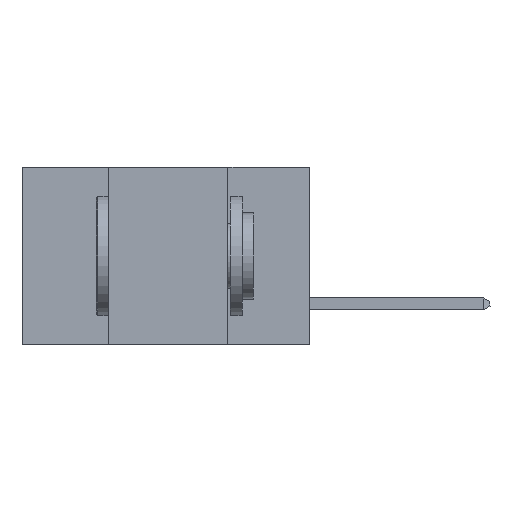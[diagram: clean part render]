
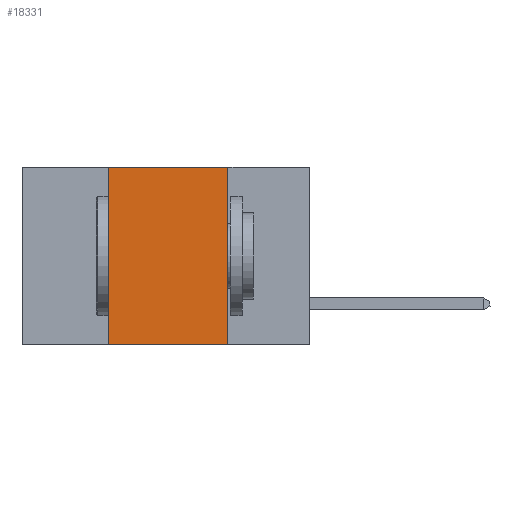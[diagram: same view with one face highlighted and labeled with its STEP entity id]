
A CAD part, left-side view. The second image highlights one B-rep face of the part: STEP entity #18331.
In plain terms, the highlighted planar face has unit normal (-1, 0, 0).
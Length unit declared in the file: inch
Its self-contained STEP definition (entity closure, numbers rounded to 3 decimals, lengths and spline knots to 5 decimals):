
#239 = VECTOR ( 'NONE', #10059, 39.37008 ) ;
#718 = VERTEX_POINT ( 'NONE', #21697 ) ;
#831 = EDGE_LOOP ( 'NONE', ( #9684, #24797, #4536, #24205 ) ) ;
#2341 = FACE_OUTER_BOUND ( 'NONE', #831, .T. ) ;
#3418 = EDGE_CURVE ( 'NONE', #30850, #718, #31739, .T. ) ;
#4372 = VECTOR ( 'NONE', #29341, 39.37008 ) ;
#4536 = ORIENTED_EDGE ( 'NONE', *, *, #8881, .F. ) ;
#5745 = CARTESIAN_POINT ( 'NONE',  ( 0., 0.42, 0. ) ) ;
#6669 = CARTESIAN_POINT ( 'NONE',  ( 0., 0.17, 0. ) ) ;
#6925 = LINE ( 'NONE', #30030, #239 ) ;
#7791 = PLANE ( 'NONE',  #30682 ) ;
#8881 = EDGE_CURVE ( 'NONE', #30850, #23092, #17730, .T. ) ;
#9241 = CARTESIAN_POINT ( 'NONE',  ( 0., 0.42, 0. ) ) ;
#9684 = ORIENTED_EDGE ( 'NONE', *, *, #11630, .F. ) ;
#10059 = DIRECTION ( 'NONE',  ( 0., 0., -1. ) ) ;
#10291 = DIRECTION ( 'NONE',  ( 1., 0., 0. ) ) ;
#11630 = EDGE_CURVE ( 'NONE', #18666, #718, #6925, .T. ) ;
#12549 = VECTOR ( 'NONE', #14240, 39.37008 ) ;
#13836 = DIRECTION ( 'NONE',  ( 0., -1., 0. ) ) ;
#14240 = DIRECTION ( 'NONE',  ( 0., -1., 0. ) ) ;
#16160 = EDGE_CURVE ( 'NONE', #23092, #18666, #17980, .T. ) ;
#17730 = LINE ( 'NONE', #9241, #4372 ) ;
#17980 = LINE ( 'NONE', #28942, #30490 ) ;
#18331 = ADVANCED_FACE ( 'NONE', ( #2341 ), #7791, .F. ) ;
#18666 = VERTEX_POINT ( 'NONE', #6669 ) ;
#21697 = CARTESIAN_POINT ( 'NONE',  ( 0., 0.17, -0.37 ) ) ;
#23092 = VERTEX_POINT ( 'NONE', #5745 ) ;
#24205 = ORIENTED_EDGE ( 'NONE', *, *, #3418, .T. ) ;
#24797 = ORIENTED_EDGE ( 'NONE', *, *, #16160, .F. ) ;
#25381 = CARTESIAN_POINT ( 'NONE',  ( 0., 0.6, 0. ) ) ;
#26843 = CARTESIAN_POINT ( 'NONE',  ( 0., 0.6, -0.37 ) ) ;
#27902 = DIRECTION ( 'NONE',  ( 0., 0., -1. ) ) ;
#28942 = CARTESIAN_POINT ( 'NONE',  ( 0., 0.6, 0. ) ) ;
#29341 = DIRECTION ( 'NONE',  ( 0., 0., 1. ) ) ;
#30030 = CARTESIAN_POINT ( 'NONE',  ( 0., 0.17, 0. ) ) ;
#30490 = VECTOR ( 'NONE', #13836, 39.37008 ) ;
#30682 = AXIS2_PLACEMENT_3D ( 'NONE', #25381, #10291, #27902 ) ;
#30850 = VERTEX_POINT ( 'NONE', #30977 ) ;
#30977 = CARTESIAN_POINT ( 'NONE',  ( 0., 0.42, -0.37 ) ) ;
#31739 = LINE ( 'NONE', #26843, #12549 ) ;
